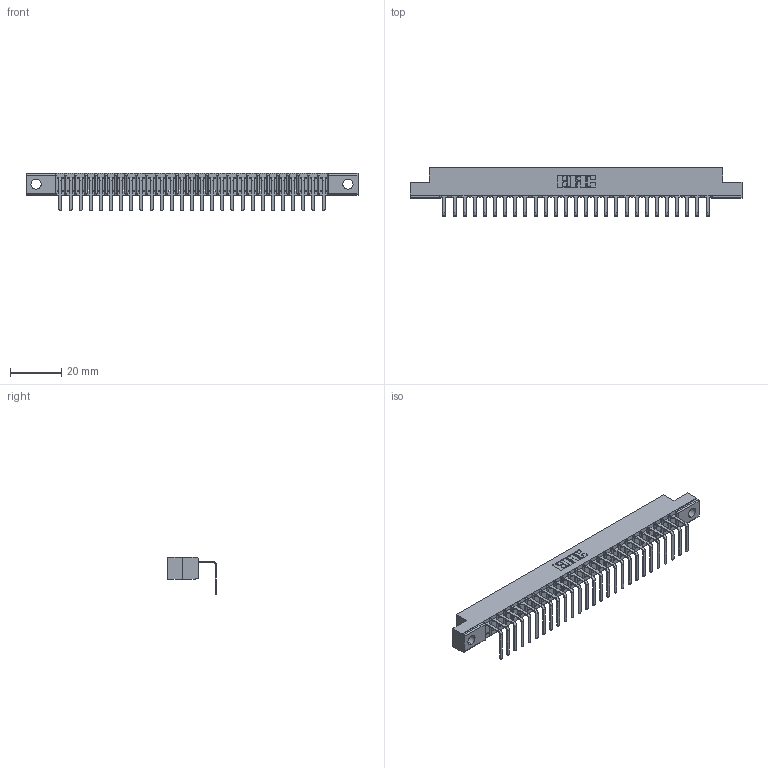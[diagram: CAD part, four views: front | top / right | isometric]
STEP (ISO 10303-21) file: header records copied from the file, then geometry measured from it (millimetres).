
FILE_DESCRIPTION (( 'STEP AP203' ), '1' );
FILE_NAME ('307-027-558-104.STEP', '2019-09-04T14:02:38', ( '' ), ( '' ), 'SwSTEP 2.0', 'SolidWorks 2016', '' );
FILE_SCHEMA (( 'CONFIG_CONTROL_DESIGN' ));
Length unit declared in the file: inch
Products named in the file (3): 307 Part_.156 Dia Mounting Holes; 307-290-001_558 - 2 (Single); 307-027-558-104
Assembly tree (28 placements, depth 2):
  307-027-558-104
    307 Part_.156 Dia Mounting Holes
    307-290-001_558 - 2 (Single)  x27
Bounding box: 130 x 18.96 x 14.81 mm (x, y, z)
Volume: 8211.5 mm3; surface area: 13530.6 mm2
Topology: 28 solids, 28 shells, 1780 faces, 5057 edges, 3258 vertices
Faces by surface type: plane 1137, cylinder 587, sphere 56
Entity records: 25518 total; most frequent: CARTESIAN_POINT 4298, ORIENTED_EDGE 4282, DIRECTION 4181, EDGE_CURVE 2141, VECTOR 1643, LINE 1643, VERTEX_POINT 1386, AXIS2_PLACEMENT_3D 1269
